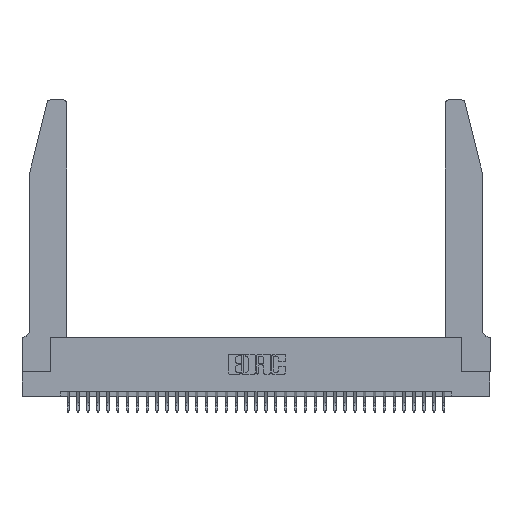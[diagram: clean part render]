
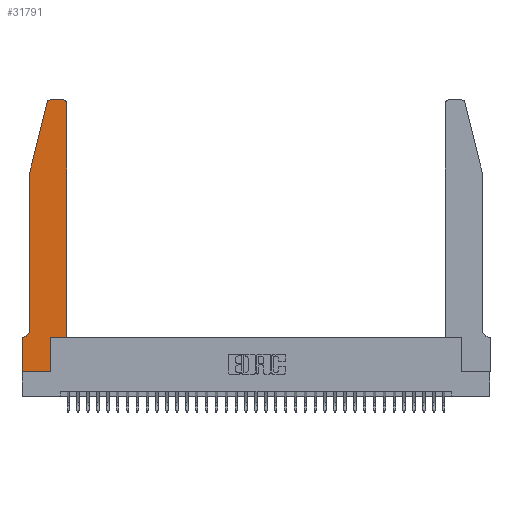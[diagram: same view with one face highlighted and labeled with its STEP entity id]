
A CAD part, top view. The second image highlights one B-rep face of the part: STEP entity #31791.
In plain terms, the highlighted planar face has unit normal (0, 0, 1).
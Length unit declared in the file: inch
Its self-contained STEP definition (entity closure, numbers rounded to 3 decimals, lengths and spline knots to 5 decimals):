
#358 = VERTEX_POINT ( 'NONE', #31001 ) ;
#637 = VECTOR ( 'NONE', #30796, 39.37008 ) ;
#1042 = VECTOR ( 'NONE', #5506, 39.37008 ) ;
#1182 = EDGE_CURVE ( 'NONE', #33998, #4501, #29682, .T. ) ;
#1572 = ORIENTED_EDGE ( 'NONE', *, *, #27773, .T. ) ;
#1602 = DIRECTION ( 'NONE',  ( -1., 0., 0. ) ) ;
#1782 = VERTEX_POINT ( 'NONE', #13467 ) ;
#2685 = CARTESIAN_POINT ( 'NONE',  ( 0.4505, 0.35, 0.37 ) ) ;
#2724 = CARTESIAN_POINT ( 'NONE',  ( 0.2865, 0.35, 0.37 ) ) ;
#3132 = CARTESIAN_POINT ( 'NONE',  ( 0.4205, 2.75, 0.37 ) ) ;
#3602 = DIRECTION ( 'NONE',  ( -1., 0., 0. ) ) ;
#4033 = ORIENTED_EDGE ( 'NONE', *, *, #1182, .T. ) ;
#4147 = ORIENTED_EDGE ( 'NONE', *, *, #25476, .T. ) ;
#4384 = CIRCLE ( 'NONE', #32411, 0.07 ) ;
#4501 = VERTEX_POINT ( 'NONE', #23312 ) ;
#5087 = EDGE_CURVE ( 'NONE', #13799, #1782, #16921, .T. ) ;
#5506 = DIRECTION ( 'NONE',  ( 0., 1., 0. ) ) ;
#5728 = ORIENTED_EDGE ( 'NONE', *, *, #20568, .T. ) ;
#5736 = CARTESIAN_POINT ( 'NONE',  ( 0.2865, 0.35, 0.37 ) ) ;
#5865 = VECTOR ( 'NONE', #6564, 39.37008 ) ;
#6564 = DIRECTION ( 'NONE',  ( 0., -1., 0. ) ) ;
#7856 = EDGE_CURVE ( 'NONE', #19212, #26542, #8909, .T. ) ;
#8049 = CARTESIAN_POINT ( 'NONE',  ( 0.0755, 2., 0.37 ) ) ;
#8195 = ORIENTED_EDGE ( 'NONE', *, *, #31393, .T. ) ;
#8509 = DIRECTION ( 'NONE',  ( 0., 0., 1. ) ) ;
#8875 = VECTOR ( 'NONE', #17777, 39.37008 ) ;
#8909 = LINE ( 'NONE', #25940, #8875 ) ;
#8959 = EDGE_CURVE ( 'NONE', #26542, #358, #9384, .T. ) ;
#9095 = ORIENTED_EDGE ( 'NONE', *, *, #19660, .T. ) ;
#9384 = LINE ( 'NONE', #2685, #1042 ) ;
#9689 = CIRCLE ( 'NONE', #11676, 0.03 ) ;
#9917 = VECTOR ( 'NONE', #21106, 39.37008 ) ;
#10839 = CARTESIAN_POINT ( 'NONE',  ( 0., 0.35, 0.37 ) ) ;
#11332 = CARTESIAN_POINT ( 'NONE',  ( 0.4205, 2.72, 0.37 ) ) ;
#11676 = AXIS2_PLACEMENT_3D ( 'NONE', #25097, #8509, #27881 ) ;
#12080 = LINE ( 'NONE', #14225, #33283 ) ;
#12957 = DIRECTION ( 'NONE',  ( 1., 0., 0. ) ) ;
#13107 = ORIENTED_EDGE ( 'NONE', *, *, #15616, .T. ) ;
#13267 = LINE ( 'NONE', #31370, #5865 ) ;
#13305 = CARTESIAN_POINT ( 'NONE',  ( 0.4505, 0.35, 0.37 ) ) ;
#13467 = CARTESIAN_POINT ( 'NONE',  ( 0.284, 2.75, 0.37 ) ) ;
#13587 = ORIENTED_EDGE ( 'NONE', *, *, #18269, .T. ) ;
#13659 = DIRECTION ( 'NONE',  ( 1., 0., 0. ) ) ;
#13799 = VERTEX_POINT ( 'NONE', #3132 ) ;
#14016 = VERTEX_POINT ( 'NONE', #29060 ) ;
#14157 = DIRECTION ( 'NONE',  ( 1., 0., 0. ) ) ;
#14225 = CARTESIAN_POINT ( 'NONE',  ( 0.0755, 0.35, 0.37 ) ) ;
#15616 = EDGE_CURVE ( 'NONE', #25007, #18207, #13267, .T. ) ;
#16921 = LINE ( 'NONE', #20272, #24264 ) ;
#17286 = LINE ( 'NONE', #5736, #637 ) ;
#17777 = DIRECTION ( 'NONE',  ( 1., 0., 0. ) ) ;
#18207 = VERTEX_POINT ( 'NONE', #28909 ) ;
#18269 = EDGE_CURVE ( 'NONE', #27212, #28547, #4384, .T. ) ;
#18327 = DIRECTION ( 'NONE',  ( 0., 0., -1. ) ) ;
#18439 = CARTESIAN_POINT ( 'NONE',  ( 0.0755, 2., 0.37 ) ) ;
#18701 = FACE_OUTER_BOUND ( 'NONE', #35164, .T. ) ;
#19212 = VERTEX_POINT ( 'NONE', #2724 ) ;
#19317 = ORIENTED_EDGE ( 'NONE', *, *, #8959, .T. ) ;
#19660 = EDGE_CURVE ( 'NONE', #4501, #27212, #32000, .T. ) ;
#19948 = DIRECTION ( 'NONE',  ( -1., 0., 0. ) ) ;
#20272 = CARTESIAN_POINT ( 'NONE',  ( 0.2605, 2.75, 0.37 ) ) ;
#20568 = EDGE_CURVE ( 'NONE', #28547, #25007, #12080, .T. ) ;
#21082 = CARTESIAN_POINT ( 'NONE',  ( 0.25487, 2.72718, 0.37 ) ) ;
#21106 = DIRECTION ( 'NONE',  ( 0., -1., 0. ) ) ;
#21327 = AXIS2_PLACEMENT_3D ( 'NONE', #11332, #30717, #14157 ) ;
#21877 = DIRECTION ( 'NONE',  ( -0.239, -0.971, 0. ) ) ;
#22025 = LINE ( 'NONE', #26745, #34943 ) ;
#22352 = VECTOR ( 'NONE', #21877, 39.37008 ) ;
#22476 = ORIENTED_EDGE ( 'NONE', *, *, #5087, .T. ) ;
#22762 = EDGE_CURVE ( 'NONE', #14016, #19212, #17286, .T. ) ;
#23312 = CARTESIAN_POINT ( 'NONE',  ( 0.0755, 2., 0.37 ) ) ;
#24264 = VECTOR ( 'NONE', #3602, 39.37008 ) ;
#25007 = VERTEX_POINT ( 'NONE', #25851 ) ;
#25097 = CARTESIAN_POINT ( 'NONE',  ( 0.284, 2.72, 0.37 ) ) ;
#25476 = EDGE_CURVE ( 'NONE', #1782, #33998, #9689, .T. ) ;
#25851 = CARTESIAN_POINT ( 'NONE',  ( 0., 0.35, 0.37 ) ) ;
#25940 = CARTESIAN_POINT ( 'NONE',  ( 0.4505, 0.35, 0.37 ) ) ;
#26143 = AXIS2_PLACEMENT_3D ( 'NONE', #10839, #30215, #13659 ) ;
#26542 = VERTEX_POINT ( 'NONE', #13305 ) ;
#26745 = CARTESIAN_POINT ( 'NONE',  ( 0., 0., 0.37 ) ) ;
#27024 = CARTESIAN_POINT ( 'NONE',  ( 0.0755, 0.42, 0.37 ) ) ;
#27212 = VERTEX_POINT ( 'NONE', #27024 ) ;
#27464 = ORIENTED_EDGE ( 'NONE', *, *, #22762, .T. ) ;
#27773 = EDGE_CURVE ( 'NONE', #18207, #14016, #22025, .T. ) ;
#27881 = DIRECTION ( 'NONE',  ( 1., 0., 0. ) ) ;
#28547 = VERTEX_POINT ( 'NONE', #35883 ) ;
#28909 = CARTESIAN_POINT ( 'NONE',  ( 0., 0., 0.37 ) ) ;
#29060 = CARTESIAN_POINT ( 'NONE',  ( 0.2865, 0., 0.37 ) ) ;
#29682 = LINE ( 'NONE', #8049, #22352 ) ;
#30100 = PLANE ( 'NONE',  #26143 ) ;
#30215 = DIRECTION ( 'NONE',  ( 0., 0., 1. ) ) ;
#30717 = DIRECTION ( 'NONE',  ( 0., 0., 1. ) ) ;
#30796 = DIRECTION ( 'NONE',  ( 0., 1., 0. ) ) ;
#31001 = CARTESIAN_POINT ( 'NONE',  ( 0.4505, 2.72, 0.37 ) ) ;
#31370 = CARTESIAN_POINT ( 'NONE',  ( 0., 0., 0.37 ) ) ;
#31393 = EDGE_CURVE ( 'NONE', #358, #13799, #35113, .T. ) ;
#31791 = ADVANCED_FACE ( 'NONE', ( #18701 ), #30100, .T. ) ;
#32000 = LINE ( 'NONE', #18439, #9917 ) ;
#32411 = AXIS2_PLACEMENT_3D ( 'NONE', #34814, #18327, #1602 ) ;
#33283 = VECTOR ( 'NONE', #19948, 39.37008 ) ;
#33998 = VERTEX_POINT ( 'NONE', #21082 ) ;
#34632 = ORIENTED_EDGE ( 'NONE', *, *, #7856, .T. ) ;
#34814 = CARTESIAN_POINT ( 'NONE',  ( 0.0055, 0.42, 0.37 ) ) ;
#34943 = VECTOR ( 'NONE', #12957, 39.37008 ) ;
#35113 = CIRCLE ( 'NONE', #21327, 0.03 ) ;
#35164 = EDGE_LOOP ( 'NONE', ( #22476, #4147, #4033, #9095, #13587, #5728, #13107, #1572, #27464, #34632, #19317, #8195 ) ) ;
#35883 = CARTESIAN_POINT ( 'NONE',  ( 0.0055, 0.35, 0.37 ) ) ;
